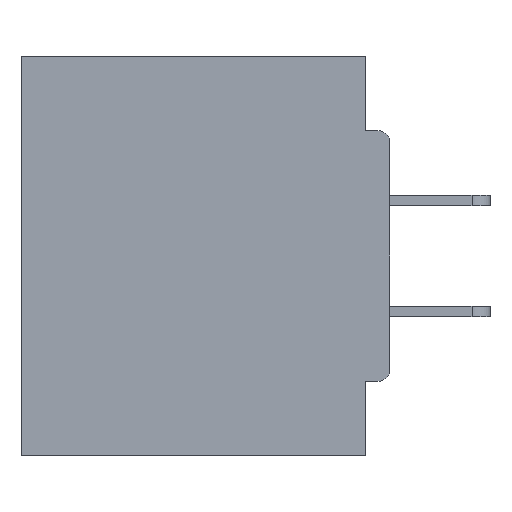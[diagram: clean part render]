
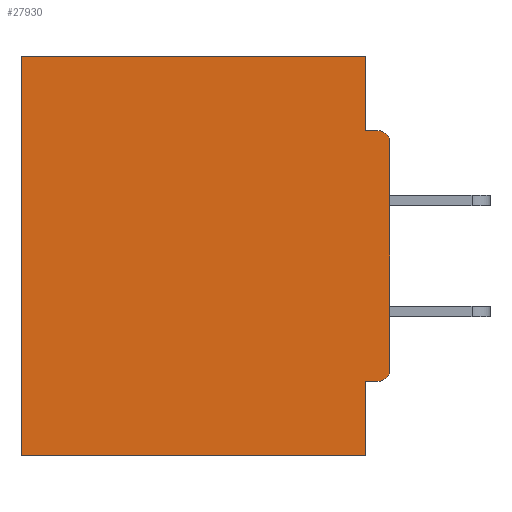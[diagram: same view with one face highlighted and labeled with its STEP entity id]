
A CAD part, left-side view. The second image highlights one B-rep face of the part: STEP entity #27930.
In plain terms, the highlighted planar face has unit normal (-1, 0, 0).
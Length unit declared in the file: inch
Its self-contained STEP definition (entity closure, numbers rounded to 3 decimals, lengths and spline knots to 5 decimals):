
#132 = DIRECTION ( 'NONE',  ( 0., 0., -1. ) ) ;
#431 = EDGE_CURVE ( 'NONE', #3699, #32938, #27694, .T. ) ;
#778 = VERTEX_POINT ( 'NONE', #28246 ) ;
#957 = LINE ( 'NONE', #23439, #29869 ) ;
#1276 = ORIENTED_EDGE ( 'NONE', *, *, #9605, .T. ) ;
#1516 = VERTEX_POINT ( 'NONE', #25559 ) ;
#3699 = VERTEX_POINT ( 'NONE', #7586 ) ;
#4752 = DIRECTION ( 'NONE',  ( -1., 0., 0. ) ) ;
#4889 = CIRCLE ( 'NONE', #7865, 0.015 ) ;
#4932 = VERTEX_POINT ( 'NONE', #20647 ) ;
#5147 = VECTOR ( 'NONE', #33875, 39.37008 ) ;
#5701 = DIRECTION ( 'NONE',  ( 0., 1., 0. ) ) ;
#5758 = AXIS2_PLACEMENT_3D ( 'NONE', #30759, #4752, #33669 ) ;
#5766 = EDGE_CURVE ( 'NONE', #4932, #778, #957, .T. ) ;
#7020 = VECTOR ( 'NONE', #22884, 39.37008 ) ;
#7586 = CARTESIAN_POINT ( 'NONE',  ( 0.298, 0.015, -0.4065 ) ) ;
#7830 = DIRECTION ( 'NONE',  ( 0., 0., -1. ) ) ;
#7838 = LINE ( 'NONE', #20459, #34015 ) ;
#7865 = AXIS2_PLACEMENT_3D ( 'NONE', #34713, #34323, #37349 ) ;
#8153 = LINE ( 'NONE', #15066, #26672 ) ;
#8202 = CARTESIAN_POINT ( 'NONE',  ( 0.298, 0.46, 0. ) ) ;
#8844 = EDGE_CURVE ( 'NONE', #4932, #29825, #37091, .T. ) ;
#9429 = EDGE_LOOP ( 'NONE', ( #27339, #16990, #33868, #28841, #1276, #26592, #10231, #27061, #23467, #30980 ) ) ;
#9556 = DIRECTION ( 'NONE',  ( 0., 1., 0. ) ) ;
#9605 = EDGE_CURVE ( 'NONE', #778, #23295, #25246, .T. ) ;
#10231 = ORIENTED_EDGE ( 'NONE', *, *, #33944, .F. ) ;
#11468 = EDGE_CURVE ( 'NONE', #3699, #16840, #11480, .T. ) ;
#11480 = CIRCLE ( 'NONE', #5758, 0.015 ) ;
#11749 = EDGE_CURVE ( 'NONE', #18439, #15321, #4889, .T. ) ;
#12378 = CARTESIAN_POINT ( 'NONE',  ( 0.298, 0.015, -0.0935 ) ) ;
#13511 = VECTOR ( 'NONE', #7830, 39.37008 ) ;
#15066 = CARTESIAN_POINT ( 'NONE',  ( 0.298, 0., -0.5 ) ) ;
#15321 = VERTEX_POINT ( 'NONE', #12378 ) ;
#15533 = LINE ( 'NONE', #25164, #5147 ) ;
#16840 = VERTEX_POINT ( 'NONE', #33788 ) ;
#16990 = ORIENTED_EDGE ( 'NONE', *, *, #34277, .F. ) ;
#17680 = CARTESIAN_POINT ( 'NONE',  ( 0.298, 0.031, -0.5 ) ) ;
#17938 = DIRECTION ( 'NONE',  ( 0., 0., -1. ) ) ;
#18439 = VERTEX_POINT ( 'NONE', #23747 ) ;
#18924 = EDGE_CURVE ( 'NONE', #18439, #16840, #7838, .T. ) ;
#20459 = CARTESIAN_POINT ( 'NONE',  ( 0.298, 0., 0. ) ) ;
#20647 = CARTESIAN_POINT ( 'NONE',  ( 0.298, 0.031, 0. ) ) ;
#20721 = AXIS2_PLACEMENT_3D ( 'NONE', #24040, #29894, #23915 ) ;
#21177 = PLANE ( 'NONE',  #20721 ) ;
#22645 = VECTOR ( 'NONE', #17938, 39.37008 ) ;
#22884 = DIRECTION ( 'NONE',  ( 0., -1., 0. ) ) ;
#23128 = CARTESIAN_POINT ( 'NONE',  ( 0.298, 0., -0.0935 ) ) ;
#23295 = VERTEX_POINT ( 'NONE', #35901 ) ;
#23439 = CARTESIAN_POINT ( 'NONE',  ( 0.298, 0., 0. ) ) ;
#23467 = ORIENTED_EDGE ( 'NONE', *, *, #11468, .T. ) ;
#23747 = CARTESIAN_POINT ( 'NONE',  ( 0.298, 0., -0.1085 ) ) ;
#23915 = DIRECTION ( 'NONE',  ( 0., 0., -1. ) ) ;
#24040 = CARTESIAN_POINT ( 'NONE',  ( 0.298, 0., 0. ) ) ;
#25164 = CARTESIAN_POINT ( 'NONE',  ( 0.298, 0.031, -0.5 ) ) ;
#25246 = LINE ( 'NONE', #8202, #13511 ) ;
#25313 = EDGE_CURVE ( 'NONE', #1516, #23295, #8153, .T. ) ;
#25559 = CARTESIAN_POINT ( 'NONE',  ( 0.298, 0.031, -0.5 ) ) ;
#26592 = ORIENTED_EDGE ( 'NONE', *, *, #25313, .F. ) ;
#26672 = VECTOR ( 'NONE', #9556, 39.37008 ) ;
#27061 = ORIENTED_EDGE ( 'NONE', *, *, #431, .F. ) ;
#27339 = ORIENTED_EDGE ( 'NONE', *, *, #11749, .T. ) ;
#27694 = LINE ( 'NONE', #29169, #36294 ) ;
#27930 = ADVANCED_FACE ( 'NONE', ( #36048 ), #21177, .F. ) ;
#28246 = CARTESIAN_POINT ( 'NONE',  ( 0.298, 0.46, 0. ) ) ;
#28841 = ORIENTED_EDGE ( 'NONE', *, *, #5766, .T. ) ;
#29169 = CARTESIAN_POINT ( 'NONE',  ( 0.298, 0., -0.4065 ) ) ;
#29825 = VERTEX_POINT ( 'NONE', #35560 ) ;
#29869 = VECTOR ( 'NONE', #34957, 39.37008 ) ;
#29894 = DIRECTION ( 'NONE',  ( 1., 0., 0. ) ) ;
#30759 = CARTESIAN_POINT ( 'NONE',  ( 0.298, 0.015, -0.3915 ) ) ;
#30980 = ORIENTED_EDGE ( 'NONE', *, *, #18924, .F. ) ;
#31849 = LINE ( 'NONE', #23128, #7020 ) ;
#32938 = VERTEX_POINT ( 'NONE', #35405 ) ;
#33669 = DIRECTION ( 'NONE',  ( 0., 0., -1. ) ) ;
#33788 = CARTESIAN_POINT ( 'NONE',  ( 0.298, 0., -0.3915 ) ) ;
#33868 = ORIENTED_EDGE ( 'NONE', *, *, #8844, .F. ) ;
#33875 = DIRECTION ( 'NONE',  ( 0., 0., -1. ) ) ;
#33944 = EDGE_CURVE ( 'NONE', #32938, #1516, #15533, .T. ) ;
#34015 = VECTOR ( 'NONE', #132, 39.37008 ) ;
#34277 = EDGE_CURVE ( 'NONE', #29825, #15321, #31849, .T. ) ;
#34323 = DIRECTION ( 'NONE',  ( -1., 0., 0. ) ) ;
#34713 = CARTESIAN_POINT ( 'NONE',  ( 0.298, 0.015, -0.1085 ) ) ;
#34957 = DIRECTION ( 'NONE',  ( 0., 1., 0. ) ) ;
#35405 = CARTESIAN_POINT ( 'NONE',  ( 0.298, 0.031, -0.4065 ) ) ;
#35560 = CARTESIAN_POINT ( 'NONE',  ( 0.298, 0.031, -0.0935 ) ) ;
#35901 = CARTESIAN_POINT ( 'NONE',  ( 0.298, 0.46, -0.5 ) ) ;
#36048 = FACE_OUTER_BOUND ( 'NONE', #9429, .T. ) ;
#36294 = VECTOR ( 'NONE', #5701, 39.37008 ) ;
#37091 = LINE ( 'NONE', #17680, #22645 ) ;
#37349 = DIRECTION ( 'NONE',  ( 0., 0., -1. ) ) ;
